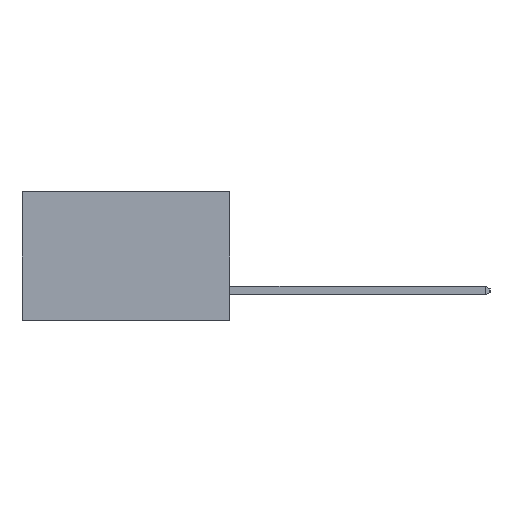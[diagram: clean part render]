
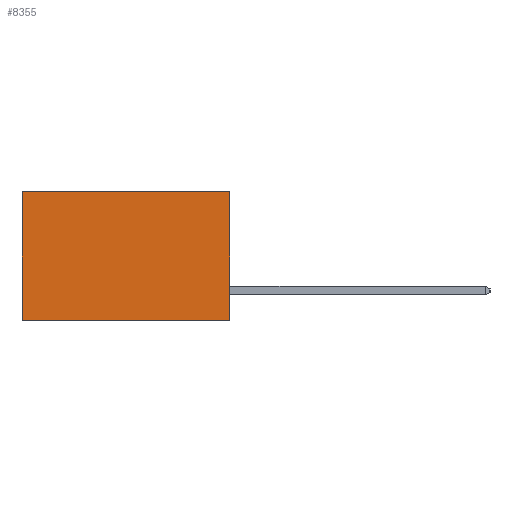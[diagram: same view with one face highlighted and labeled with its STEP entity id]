
A CAD part, left-side view. The second image highlights one B-rep face of the part: STEP entity #8355.
In plain terms, the highlighted planar face has unit normal (-1, 0, 0).
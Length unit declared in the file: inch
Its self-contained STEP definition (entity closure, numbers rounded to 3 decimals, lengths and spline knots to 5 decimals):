
#158 = FACE_OUTER_BOUND ( 'NONE', #4653, .T. ) ;
#608 = ORIENTED_EDGE ( 'NONE', *, *, #5855, .T. ) ;
#1038 = VERTEX_POINT ( 'NONE', #7698 ) ;
#1485 = LINE ( 'NONE', #2136, #13115 ) ;
#1494 = DIRECTION ( 'NONE',  ( 0., 0., -1. ) ) ;
#1793 = VERTEX_POINT ( 'NONE', #13296 ) ;
#1836 = VECTOR ( 'NONE', #11321, 39.37008 ) ;
#2136 = CARTESIAN_POINT ( 'NONE',  ( 0.2615, 0., 0. ) ) ;
#2634 = EDGE_CURVE ( 'NONE', #5574, #1793, #10329, .T. ) ;
#4653 = EDGE_LOOP ( 'NONE', ( #608, #8624, #9525, #11845 ) ) ;
#4802 = CARTESIAN_POINT ( 'NONE',  ( 0.2615, 0., 0. ) ) ;
#4875 = CARTESIAN_POINT ( 'NONE',  ( 0.2615, 0., -0.37 ) ) ;
#4967 = CARTESIAN_POINT ( 'NONE',  ( 0.2615, 0., -0.37 ) ) ;
#5020 = AXIS2_PLACEMENT_3D ( 'NONE', #4875, #5375, #5897 ) ;
#5190 = VERTEX_POINT ( 'NONE', #4802 ) ;
#5375 = DIRECTION ( 'NONE',  ( 1., 0., 0. ) ) ;
#5527 = PLANE ( 'NONE',  #5020 ) ;
#5574 = VERTEX_POINT ( 'NONE', #13237 ) ;
#5841 = VECTOR ( 'NONE', #1494, 39.37008 ) ;
#5855 = EDGE_CURVE ( 'NONE', #1038, #1793, #8218, .T. ) ;
#5897 = DIRECTION ( 'NONE',  ( 0., 0., -1. ) ) ;
#7698 = CARTESIAN_POINT ( 'NONE',  ( 0.2615, 0.6, 0. ) ) ;
#7780 = DIRECTION ( 'NONE',  ( 0., 1., 0. ) ) ;
#8218 = LINE ( 'NONE', #11297, #1836 ) ;
#8355 = ADVANCED_FACE ( 'NONE', ( #158 ), #5527, .F. ) ;
#8417 = LINE ( 'NONE', #4967, #5841 ) ;
#8624 = ORIENTED_EDGE ( 'NONE', *, *, #2634, .F. ) ;
#9156 = DIRECTION ( 'NONE',  ( 0., 1., 0. ) ) ;
#9525 = ORIENTED_EDGE ( 'NONE', *, *, #10605, .F. ) ;
#10329 = LINE ( 'NONE', #13192, #13095 ) ;
#10605 = EDGE_CURVE ( 'NONE', #5190, #5574, #8417, .T. ) ;
#11297 = CARTESIAN_POINT ( 'NONE',  ( 0.2615, 0.6, -0.37 ) ) ;
#11321 = DIRECTION ( 'NONE',  ( 0., 0., -1. ) ) ;
#11845 = ORIENTED_EDGE ( 'NONE', *, *, #14002, .T. ) ;
#13095 = VECTOR ( 'NONE', #9156, 39.37008 ) ;
#13115 = VECTOR ( 'NONE', #7780, 39.37008 ) ;
#13192 = CARTESIAN_POINT ( 'NONE',  ( 0.2615, 0., -0.37 ) ) ;
#13237 = CARTESIAN_POINT ( 'NONE',  ( 0.2615, 0., -0.37 ) ) ;
#13296 = CARTESIAN_POINT ( 'NONE',  ( 0.2615, 0.6, -0.37 ) ) ;
#14002 = EDGE_CURVE ( 'NONE', #5190, #1038, #1485, .T. ) ;
